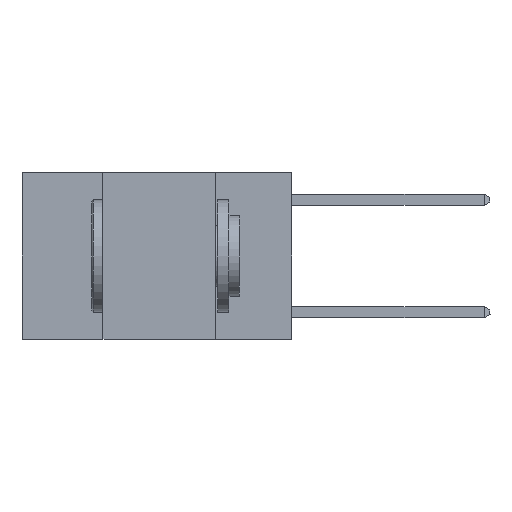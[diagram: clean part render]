
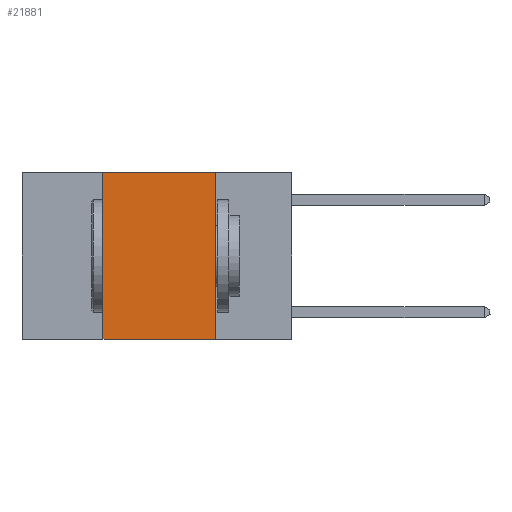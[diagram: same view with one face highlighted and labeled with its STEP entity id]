
A CAD part, left-side view. The second image highlights one B-rep face of the part: STEP entity #21881.
In plain terms, the highlighted planar face has unit normal (-1, 0, 0).
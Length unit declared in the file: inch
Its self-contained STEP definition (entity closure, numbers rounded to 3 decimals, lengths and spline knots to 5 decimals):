
#573 = DIRECTION ( 'NONE',  ( 0., -1., 0. ) ) ;
#2059 = DIRECTION ( 'NONE',  ( 0., 0., -1. ) ) ;
#2071 = EDGE_CURVE ( 'NONE', #7179, #19391, #7493, .T. ) ;
#3340 = EDGE_CURVE ( 'NONE', #18413, #7179, #13831, .T. ) ;
#3773 = CARTESIAN_POINT ( 'NONE',  ( 0., 0.42, 0. ) ) ;
#3987 = CARTESIAN_POINT ( 'NONE',  ( 0., 0.17, 0. ) ) ;
#5626 = DIRECTION ( 'NONE',  ( 0., 0., 1. ) ) ;
#5741 = VECTOR ( 'NONE', #23028, 39.37008 ) ;
#6375 = CARTESIAN_POINT ( 'NONE',  ( 0., 0.42, 0. ) ) ;
#6542 = CARTESIAN_POINT ( 'NONE',  ( 0., 0.42, -0.37 ) ) ;
#6679 = LINE ( 'NONE', #21080, #9832 ) ;
#6751 = EDGE_CURVE ( 'NONE', #18413, #23030, #19446, .T. ) ;
#7179 = VERTEX_POINT ( 'NONE', #6375 ) ;
#7493 = LINE ( 'NONE', #21929, #16960 ) ;
#8862 = DIRECTION ( 'NONE',  ( 0., 0., -1. ) ) ;
#9832 = VECTOR ( 'NONE', #8862, 39.37008 ) ;
#9885 = AXIS2_PLACEMENT_3D ( 'NONE', #12830, #12905, #2059 ) ;
#11288 = ORIENTED_EDGE ( 'NONE', *, *, #19126, .F. ) ;
#11647 = ORIENTED_EDGE ( 'NONE', *, *, #2071, .F. ) ;
#11906 = FACE_OUTER_BOUND ( 'NONE', #12505, .T. ) ;
#11993 = ORIENTED_EDGE ( 'NONE', *, *, #3340, .F. ) ;
#12136 = ORIENTED_EDGE ( 'NONE', *, *, #6751, .T. ) ;
#12505 = EDGE_LOOP ( 'NONE', ( #11288, #11647, #11993, #12136 ) ) ;
#12830 = CARTESIAN_POINT ( 'NONE',  ( 0., 0.6, 0. ) ) ;
#12905 = DIRECTION ( 'NONE',  ( 1., 0., 0. ) ) ;
#13831 = LINE ( 'NONE', #3773, #22494 ) ;
#16960 = VECTOR ( 'NONE', #573, 39.37008 ) ;
#17916 = CARTESIAN_POINT ( 'NONE',  ( 0., 0.6, -0.37 ) ) ;
#18413 = VERTEX_POINT ( 'NONE', #6542 ) ;
#19126 = EDGE_CURVE ( 'NONE', #19391, #23030, #6679, .T. ) ;
#19391 = VERTEX_POINT ( 'NONE', #3987 ) ;
#19446 = LINE ( 'NONE', #17916, #5741 ) ;
#19952 = PLANE ( 'NONE',  #9885 ) ;
#21080 = CARTESIAN_POINT ( 'NONE',  ( 0., 0.17, 0. ) ) ;
#21748 = CARTESIAN_POINT ( 'NONE',  ( 0., 0.17, -0.37 ) ) ;
#21881 = ADVANCED_FACE ( 'NONE', ( #11906 ), #19952, .F. ) ;
#21929 = CARTESIAN_POINT ( 'NONE',  ( 0., 0.6, 0. ) ) ;
#22494 = VECTOR ( 'NONE', #5626, 39.37008 ) ;
#23028 = DIRECTION ( 'NONE',  ( 0., -1., 0. ) ) ;
#23030 = VERTEX_POINT ( 'NONE', #21748 ) ;
